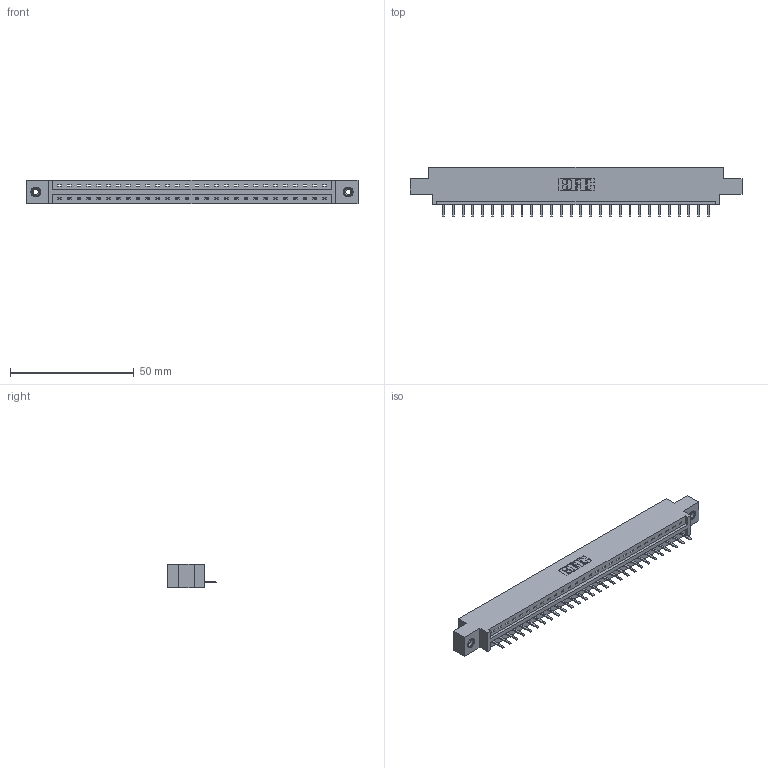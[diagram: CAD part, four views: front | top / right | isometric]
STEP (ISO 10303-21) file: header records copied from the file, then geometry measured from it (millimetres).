
FILE_DESCRIPTION (( 'STEP AP203' ), '1' );
FILE_NAME ('387-028-520-608.STEP', '2019-10-03T14:34:46', ( '' ), ( '' ), 'SwSTEP 2.0', 'SolidWorks 2016', '' );
FILE_SCHEMA (( 'CONFIG_CONTROL_DESIGN' ));
Length unit declared in the file: inch
Products named in the file (4): 345-292-001_345-293-120; 387-028-520-608; 345-250-001_345-250-003-102; 337 Part_0.170 Offset - 0.156 Dia-TI
Assembly tree (31 placements, depth 2):
  387-028-520-608
    337 Part_0.170 Offset - 0.156 Dia-TI
    345-292-001_345-293-120  x28
    345-250-001_345-250-003-102  x2
Bounding box: 133.96 x 20.02 x 9.4 mm (x, y, z)
Volume: 13543.1 mm3; surface area: 13753.3 mm2
Topology: 31 solids, 31 shells, 2026 faces, 5947 edges, 3882 vertices
Faces by surface type: plane 1450, cylinder 560, cone 12, torus 4
Entity records: 24056 total; most frequent: CARTESIAN_POINT 4181, ORIENTED_EDGE 4126, DIRECTION 3569, EDGE_CURVE 2063, VECTOR 1911, LINE 1911, VERTEX_POINT 1368, AXIS2_PLACEMENT_3D 829
